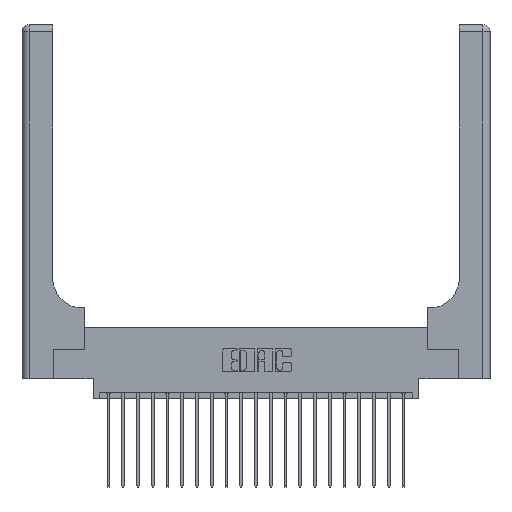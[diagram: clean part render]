
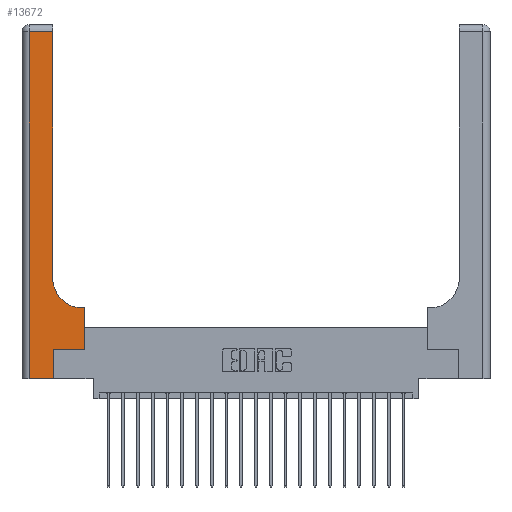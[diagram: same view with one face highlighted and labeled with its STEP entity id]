
A CAD part, top view. The second image highlights one B-rep face of the part: STEP entity #13672.
In plain terms, the highlighted planar face has unit normal (0, 0, 1).
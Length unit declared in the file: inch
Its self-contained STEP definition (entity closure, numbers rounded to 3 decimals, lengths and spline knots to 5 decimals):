
#227 = VECTOR ( 'NONE', #2950, 39.37008 ) ;
#505 = ORIENTED_EDGE ( 'NONE', *, *, #20929, .T. ) ;
#805 = LINE ( 'NONE', #18504, #18298 ) ;
#1199 = ORIENTED_EDGE ( 'NONE', *, *, #21530, .T. ) ;
#1669 = VERTEX_POINT ( 'NONE', #13032 ) ;
#1714 = VERTEX_POINT ( 'NONE', #18161 ) ;
#2514 = ORIENTED_EDGE ( 'NONE', *, *, #14379, .T. ) ;
#2950 = DIRECTION ( 'NONE',  ( 1., 0., 0. ) ) ;
#3030 = DIRECTION ( 'NONE',  ( 0., -1., 0. ) ) ;
#3050 = ORIENTED_EDGE ( 'NONE', *, *, #10079, .T. ) ;
#3516 = CARTESIAN_POINT ( 'NONE',  ( 0., 2.94, 0.37 ) ) ;
#3784 = EDGE_CURVE ( 'NONE', #10758, #1714, #8007, .T. ) ;
#4235 = LINE ( 'NONE', #14112, #21086 ) ;
#4475 = VERTEX_POINT ( 'NONE', #5348 ) ;
#4546 = VECTOR ( 'NONE', #5231, 39.37008 ) ;
#4818 = PLANE ( 'NONE',  #18348 ) ;
#4853 = EDGE_CURVE ( 'NONE', #4475, #7005, #9876, .T. ) ;
#5231 = DIRECTION ( 'NONE',  ( -1., 0., 0. ) ) ;
#5257 = VERTEX_POINT ( 'NONE', #7478 ) ;
#5342 = DIRECTION ( 'NONE',  ( 0., 0., -1. ) ) ;
#5348 = CARTESIAN_POINT ( 'NONE',  ( 0.06, 0., 0.37 ) ) ;
#5542 = CARTESIAN_POINT ( 'NONE',  ( 0.528, 0.25, 0.37 ) ) ;
#5731 = LINE ( 'NONE', #5542, #14260 ) ;
#5842 = CIRCLE ( 'NONE', #20848, 0.25 ) ;
#6497 = EDGE_CURVE ( 'NONE', #16751, #1669, #5842, .T. ) ;
#7005 = VERTEX_POINT ( 'NONE', #8457 ) ;
#7478 = CARTESIAN_POINT ( 'NONE',  ( 0.265, 0.25, 0.37 ) ) ;
#8007 = LINE ( 'NONE', #3516, #4546 ) ;
#8245 = DIRECTION ( 'NONE',  ( -1., 0., 0. ) ) ;
#8457 = CARTESIAN_POINT ( 'NONE',  ( 0.265, 0., 0.37 ) ) ;
#8926 = ORIENTED_EDGE ( 'NONE', *, *, #6497, .T. ) ;
#9876 = LINE ( 'NONE', #14878, #227 ) ;
#10079 = EDGE_CURVE ( 'NONE', #5257, #19939, #11581, .T. ) ;
#10281 = VECTOR ( 'NONE', #21592, 39.37008 ) ;
#10758 = VERTEX_POINT ( 'NONE', #13640 ) ;
#10829 = LINE ( 'NONE', #18236, #10281 ) ;
#10981 = VECTOR ( 'NONE', #3030, 39.37008 ) ;
#11040 = CARTESIAN_POINT ( 'NONE',  ( 0.265, 0.25, 0.37 ) ) ;
#11581 = LINE ( 'NONE', #11040, #19908 ) ;
#13032 = CARTESIAN_POINT ( 'NONE',  ( 0.26, 0.85, 0.37 ) ) ;
#13044 = CARTESIAN_POINT ( 'NONE',  ( 0.51, 0.6, 0.37 ) ) ;
#13274 = CARTESIAN_POINT ( 'NONE',  ( 0.06, 3., 0.37 ) ) ;
#13626 = EDGE_CURVE ( 'NONE', #1714, #4475, #14973, .T. ) ;
#13640 = CARTESIAN_POINT ( 'NONE',  ( 0.26, 2.94, 0.37 ) ) ;
#13672 = ADVANCED_FACE ( 'NONE', ( #17771 ), #4818, .F. ) ;
#14103 = ORIENTED_EDGE ( 'NONE', *, *, #15981, .T. ) ;
#14112 = CARTESIAN_POINT ( 'NONE',  ( 0.26, 0.6, 0.37 ) ) ;
#14260 = VECTOR ( 'NONE', #17358, 39.37008 ) ;
#14379 = EDGE_CURVE ( 'NONE', #7005, #5257, #805, .T. ) ;
#14878 = CARTESIAN_POINT ( 'NONE',  ( 0., 0., 0.37 ) ) ;
#14973 = LINE ( 'NONE', #13274, #10981 ) ;
#15216 = DIRECTION ( 'NONE',  ( 0., 1., 0. ) ) ;
#15534 = CARTESIAN_POINT ( 'NONE',  ( 0.51, 0.85, 0.37 ) ) ;
#15566 = CARTESIAN_POINT ( 'NONE',  ( 0.528, 0.25, 0.37 ) ) ;
#15789 = DIRECTION ( 'NONE',  ( -1., 0., 0. ) ) ;
#15981 = EDGE_CURVE ( 'NONE', #20375, #16751, #4235, .T. ) ;
#16063 = DIRECTION ( 'NONE',  ( 1., 0., 0. ) ) ;
#16422 = EDGE_LOOP ( 'NONE', ( #505, #17913, #16583, #18064, #2514, #3050, #1199, #14103, #8926 ) ) ;
#16583 = ORIENTED_EDGE ( 'NONE', *, *, #13626, .T. ) ;
#16682 = CARTESIAN_POINT ( 'NONE',  ( 0., 3., 0.37 ) ) ;
#16751 = VERTEX_POINT ( 'NONE', #13044 ) ;
#16907 = CARTESIAN_POINT ( 'NONE',  ( 0.528, 0.6, 0.37 ) ) ;
#17187 = DIRECTION ( 'NONE',  ( 1., 0., 0. ) ) ;
#17358 = DIRECTION ( 'NONE',  ( 0., 1., 0. ) ) ;
#17771 = FACE_OUTER_BOUND ( 'NONE', #16422, .T. ) ;
#17913 = ORIENTED_EDGE ( 'NONE', *, *, #3784, .T. ) ;
#18064 = ORIENTED_EDGE ( 'NONE', *, *, #4853, .T. ) ;
#18161 = CARTESIAN_POINT ( 'NONE',  ( 0.06, 2.94, 0.37 ) ) ;
#18236 = CARTESIAN_POINT ( 'NONE',  ( 0.26, 3., 0.37 ) ) ;
#18298 = VECTOR ( 'NONE', #15216, 39.37008 ) ;
#18324 = DIRECTION ( 'NONE',  ( 0., 0., -1. ) ) ;
#18348 = AXIS2_PLACEMENT_3D ( 'NONE', #16682, #18324, #8245 ) ;
#18504 = CARTESIAN_POINT ( 'NONE',  ( 0.265, 0., 0.37 ) ) ;
#19908 = VECTOR ( 'NONE', #16063, 39.37008 ) ;
#19939 = VERTEX_POINT ( 'NONE', #15566 ) ;
#20375 = VERTEX_POINT ( 'NONE', #16907 ) ;
#20848 = AXIS2_PLACEMENT_3D ( 'NONE', #15534, #5342, #17187 ) ;
#20929 = EDGE_CURVE ( 'NONE', #1669, #10758, #10829, .T. ) ;
#21086 = VECTOR ( 'NONE', #15789, 39.37008 ) ;
#21530 = EDGE_CURVE ( 'NONE', #19939, #20375, #5731, .T. ) ;
#21592 = DIRECTION ( 'NONE',  ( 0., 1., 0. ) ) ;
